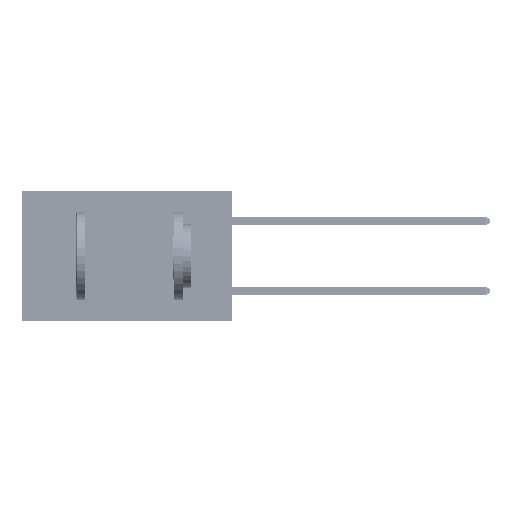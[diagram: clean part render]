
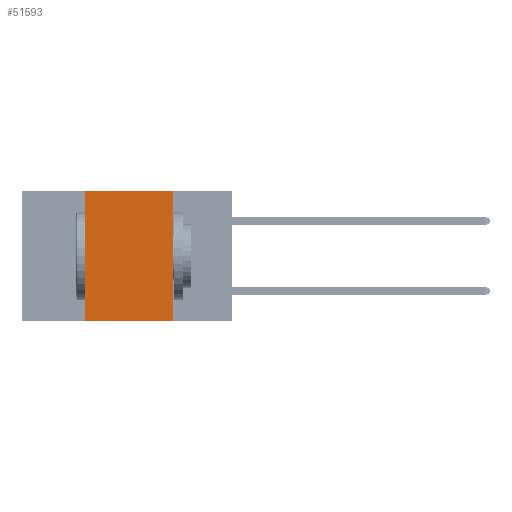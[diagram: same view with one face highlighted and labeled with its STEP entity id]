
A CAD part, left-side view. The second image highlights one B-rep face of the part: STEP entity #51593.
In plain terms, the highlighted planar face has unit normal (-1, 0, 0).
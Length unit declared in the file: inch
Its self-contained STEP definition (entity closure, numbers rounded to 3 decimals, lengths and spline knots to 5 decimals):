
#6322 = VERTEX_POINT ( 'NONE', #16052 ) ;
#6511 = VERTEX_POINT ( 'NONE', #36786 ) ;
#6550 = EDGE_CURVE ( 'NONE', #6322, #30148, #14243, .T. ) ;
#6621 = ORIENTED_EDGE ( 'NONE', *, *, #17623, .T. ) ;
#7070 = AXIS2_PLACEMENT_3D ( 'NONE', #49133, #16502, #11721 ) ;
#8957 = DIRECTION ( 'NONE',  ( 0., -1., 0. ) ) ;
#11721 = DIRECTION ( 'NONE',  ( 0., 0., -1. ) ) ;
#12360 = EDGE_CURVE ( 'NONE', #6511, #6322, #50034, .T. ) ;
#12410 = PLANE ( 'NONE',  #7070 ) ;
#14243 = LINE ( 'NONE', #29089, #27026 ) ;
#16052 = CARTESIAN_POINT ( 'NONE',  ( 0., 0.17, 0. ) ) ;
#16502 = DIRECTION ( 'NONE',  ( 1., 0., 0. ) ) ;
#17623 = EDGE_CURVE ( 'NONE', #46822, #30148, #51746, .T. ) ;
#20460 = ORIENTED_EDGE ( 'NONE', *, *, #6550, .F. ) ;
#24766 = ORIENTED_EDGE ( 'NONE', *, *, #41359, .F. ) ;
#25907 = ORIENTED_EDGE ( 'NONE', *, *, #12360, .F. ) ;
#27026 = VECTOR ( 'NONE', #44873, 39.37008 ) ;
#29089 = CARTESIAN_POINT ( 'NONE',  ( 0., 0.17, 0. ) ) ;
#29203 = CARTESIAN_POINT ( 'NONE',  ( 0., 0.42, -0.37 ) ) ;
#29335 = CARTESIAN_POINT ( 'NONE',  ( 0., 0.6, 0. ) ) ;
#29492 = DIRECTION ( 'NONE',  ( 0., 0., 1. ) ) ;
#29509 = VECTOR ( 'NONE', #8957, 39.37008 ) ;
#30148 = VERTEX_POINT ( 'NONE', #47367 ) ;
#31092 = CARTESIAN_POINT ( 'NONE',  ( 0., 0.6, -0.37 ) ) ;
#31162 = LINE ( 'NONE', #49744, #44632 ) ;
#35039 = DIRECTION ( 'NONE',  ( 0., -1., 0. ) ) ;
#36786 = CARTESIAN_POINT ( 'NONE',  ( 0., 0.42, 0. ) ) ;
#36939 = VECTOR ( 'NONE', #35039, 39.37008 ) ;
#41359 = EDGE_CURVE ( 'NONE', #46822, #6511, #31162, .T. ) ;
#41559 = EDGE_LOOP ( 'NONE', ( #20460, #25907, #24766, #6621 ) ) ;
#43490 = FACE_OUTER_BOUND ( 'NONE', #41559, .T. ) ;
#44632 = VECTOR ( 'NONE', #29492, 39.37008 ) ;
#44873 = DIRECTION ( 'NONE',  ( 0., 0., -1. ) ) ;
#46822 = VERTEX_POINT ( 'NONE', #29203 ) ;
#47367 = CARTESIAN_POINT ( 'NONE',  ( 0., 0.17, -0.37 ) ) ;
#49133 = CARTESIAN_POINT ( 'NONE',  ( 0., 0.6, 0. ) ) ;
#49744 = CARTESIAN_POINT ( 'NONE',  ( 0., 0.42, 0. ) ) ;
#50034 = LINE ( 'NONE', #29335, #29509 ) ;
#51593 = ADVANCED_FACE ( 'NONE', ( #43490 ), #12410, .F. ) ;
#51746 = LINE ( 'NONE', #31092, #36939 ) ;
